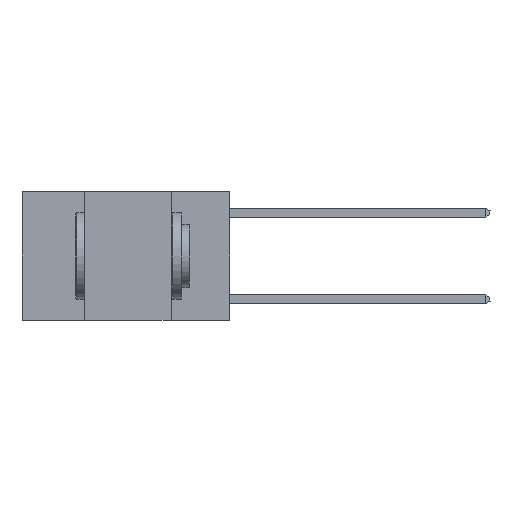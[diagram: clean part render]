
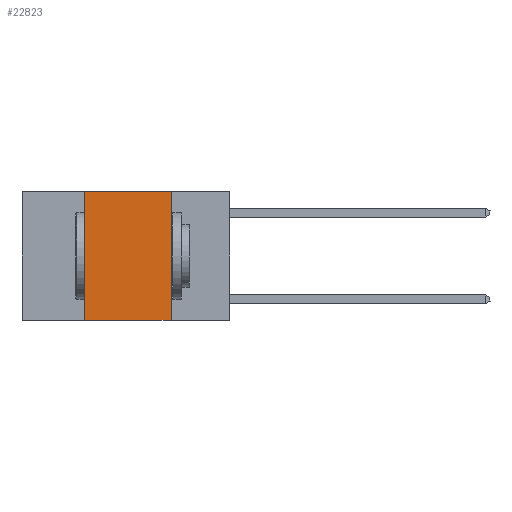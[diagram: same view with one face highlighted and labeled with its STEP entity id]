
A CAD part, left-side view. The second image highlights one B-rep face of the part: STEP entity #22823.
In plain terms, the highlighted planar face has unit normal (-1, 0, 0).
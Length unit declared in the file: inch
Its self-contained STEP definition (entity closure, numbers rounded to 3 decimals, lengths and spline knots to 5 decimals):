
#151 = ORIENTED_EDGE ( 'NONE', *, *, #7359, .F. ) ;
#1783 = ORIENTED_EDGE ( 'NONE', *, *, #10527, .T. ) ;
#1807 = LINE ( 'NONE', #12928, #19774 ) ;
#4368 = CARTESIAN_POINT ( 'NONE',  ( 0., 0.6, -0.37 ) ) ;
#4953 = DIRECTION ( 'NONE',  ( 0., 0., -1. ) ) ;
#5459 = EDGE_CURVE ( 'NONE', #10591, #16557, #22643, .T. ) ;
#5703 = VERTEX_POINT ( 'NONE', #29575 ) ;
#5810 = AXIS2_PLACEMENT_3D ( 'NONE', #24226, #26569, #12571 ) ;
#7359 = EDGE_CURVE ( 'NONE', #29119, #10591, #1807, .T. ) ;
#7867 = PLANE ( 'NONE',  #5810 ) ;
#7936 = LINE ( 'NONE', #16636, #13433 ) ;
#9100 = DIRECTION ( 'NONE',  ( 0., -1., 0. ) ) ;
#9306 = CARTESIAN_POINT ( 'NONE',  ( 0., 0.42, 0. ) ) ;
#10206 = VECTOR ( 'NONE', #28785, 39.37008 ) ;
#10527 = EDGE_CURVE ( 'NONE', #29119, #5703, #22970, .T. ) ;
#10536 = VECTOR ( 'NONE', #9100, 39.37008 ) ;
#10591 = VERTEX_POINT ( 'NONE', #9306 ) ;
#12465 = CARTESIAN_POINT ( 'NONE',  ( 0., 0.6, 0. ) ) ;
#12571 = DIRECTION ( 'NONE',  ( 0., 0., -1. ) ) ;
#12638 = ORIENTED_EDGE ( 'NONE', *, *, #5459, .F. ) ;
#12928 = CARTESIAN_POINT ( 'NONE',  ( 0., 0.42, 0. ) ) ;
#13433 = VECTOR ( 'NONE', #4953, 39.37008 ) ;
#14342 = EDGE_LOOP ( 'NONE', ( #22696, #12638, #151, #1783 ) ) ;
#16557 = VERTEX_POINT ( 'NONE', #17031 ) ;
#16636 = CARTESIAN_POINT ( 'NONE',  ( 0., 0.17, 0. ) ) ;
#17031 = CARTESIAN_POINT ( 'NONE',  ( 0., 0.17, 0. ) ) ;
#18351 = EDGE_CURVE ( 'NONE', #16557, #5703, #7936, .T. ) ;
#18401 = FACE_OUTER_BOUND ( 'NONE', #14342, .T. ) ;
#19774 = VECTOR ( 'NONE', #29239, 39.37008 ) ;
#22643 = LINE ( 'NONE', #12465, #10206 ) ;
#22696 = ORIENTED_EDGE ( 'NONE', *, *, #18351, .F. ) ;
#22823 = ADVANCED_FACE ( 'NONE', ( #18401 ), #7867, .F. ) ;
#22970 = LINE ( 'NONE', #4368, #10536 ) ;
#24226 = CARTESIAN_POINT ( 'NONE',  ( 0., 0.6, 0. ) ) ;
#26569 = DIRECTION ( 'NONE',  ( 1., 0., 0. ) ) ;
#28785 = DIRECTION ( 'NONE',  ( 0., -1., 0. ) ) ;
#29119 = VERTEX_POINT ( 'NONE', #29130 ) ;
#29130 = CARTESIAN_POINT ( 'NONE',  ( 0., 0.42, -0.37 ) ) ;
#29239 = DIRECTION ( 'NONE',  ( 0., 0., 1. ) ) ;
#29575 = CARTESIAN_POINT ( 'NONE',  ( 0., 0.17, -0.37 ) ) ;
